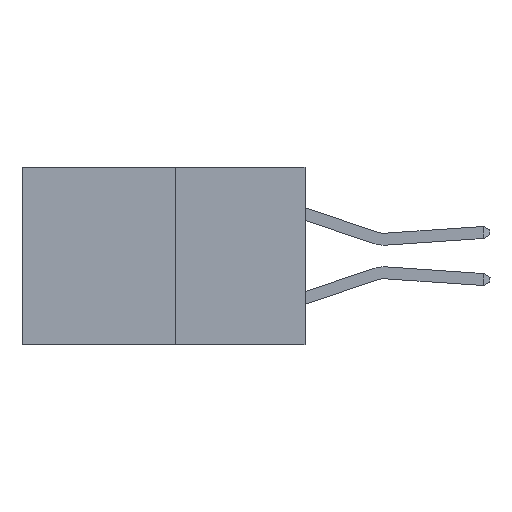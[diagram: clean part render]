
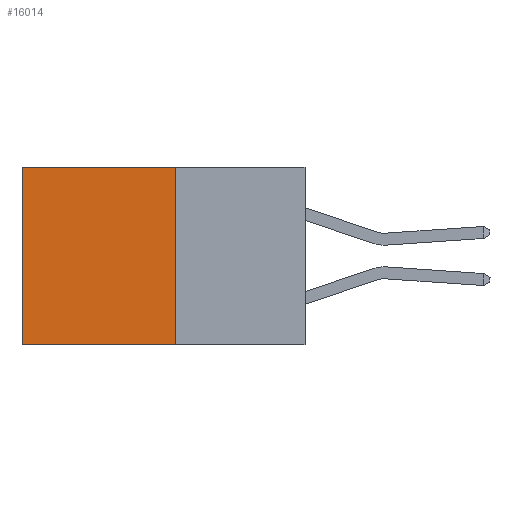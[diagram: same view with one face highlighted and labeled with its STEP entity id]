
A CAD part, left-side view. The second image highlights one B-rep face of the part: STEP entity #16014.
In plain terms, the highlighted planar face has unit normal (-1, 0, 0).
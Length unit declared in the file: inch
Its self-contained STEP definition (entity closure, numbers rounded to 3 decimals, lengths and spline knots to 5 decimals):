
#1238 = EDGE_LOOP ( 'NONE', ( #16327, #9316, #17948, #20871 ) ) ;
#1451 = PLANE ( 'NONE',  #13199 ) ;
#2006 = CARTESIAN_POINT ( 'NONE',  ( 0.277, 0.27, 0. ) ) ;
#3659 = CARTESIAN_POINT ( 'NONE',  ( 0.277, 0.27, 0. ) ) ;
#4166 = DIRECTION ( 'NONE',  ( 0., 1., 0. ) ) ;
#5233 = EDGE_CURVE ( 'NONE', #19410, #13453, #23947, .T. ) ;
#5755 = DIRECTION ( 'NONE',  ( 0., 1., 0. ) ) ;
#5861 = CARTESIAN_POINT ( 'NONE',  ( 0.277, 0.59, 0. ) ) ;
#6057 = CARTESIAN_POINT ( 'NONE',  ( 0.277, 0.27, -0.37 ) ) ;
#8040 = VECTOR ( 'NONE', #5755, 39.37008 ) ;
#9316 = ORIENTED_EDGE ( 'NONE', *, *, #25436, .F. ) ;
#9379 = DIRECTION ( 'NONE',  ( 0., 0., -1. ) ) ;
#9954 = VERTEX_POINT ( 'NONE', #2006 ) ;
#9957 = CARTESIAN_POINT ( 'NONE',  ( 0.277, 0.59, -0.37 ) ) ;
#10355 = CARTESIAN_POINT ( 'NONE',  ( 0.277, 0.27, -0.37 ) ) ;
#11150 = VERTEX_POINT ( 'NONE', #15870 ) ;
#13199 = AXIS2_PLACEMENT_3D ( 'NONE', #22018, #26175, #13968 ) ;
#13453 = VERTEX_POINT ( 'NONE', #15407 ) ;
#13968 = DIRECTION ( 'NONE',  ( 0., 0., -1. ) ) ;
#15407 = CARTESIAN_POINT ( 'NONE',  ( 0.277, 0.59, -0.37 ) ) ;
#15466 = VECTOR ( 'NONE', #18342, 39.37008 ) ;
#15870 = CARTESIAN_POINT ( 'NONE',  ( 0.277, 0.27, -0.37 ) ) ;
#16014 = ADVANCED_FACE ( 'NONE', ( #16869 ), #1451, .F. ) ;
#16327 = ORIENTED_EDGE ( 'NONE', *, *, #5233, .T. ) ;
#16869 = FACE_OUTER_BOUND ( 'NONE', #1238, .T. ) ;
#17948 = ORIENTED_EDGE ( 'NONE', *, *, #22401, .F. ) ;
#18342 = DIRECTION ( 'NONE',  ( 0., 0., -1. ) ) ;
#18517 = VECTOR ( 'NONE', #9379, 39.37008 ) ;
#18964 = LINE ( 'NONE', #10355, #23100 ) ;
#19410 = VERTEX_POINT ( 'NONE', #5861 ) ;
#20871 = ORIENTED_EDGE ( 'NONE', *, *, #22985, .T. ) ;
#22018 = CARTESIAN_POINT ( 'NONE',  ( 0.277, 0.27, -0.37 ) ) ;
#22401 = EDGE_CURVE ( 'NONE', #9954, #11150, #26293, .T. ) ;
#22985 = EDGE_CURVE ( 'NONE', #9954, #19410, #23694, .T. ) ;
#23100 = VECTOR ( 'NONE', #4166, 39.37008 ) ;
#23694 = LINE ( 'NONE', #3659, #8040 ) ;
#23947 = LINE ( 'NONE', #9957, #18517 ) ;
#25436 = EDGE_CURVE ( 'NONE', #11150, #13453, #18964, .T. ) ;
#26175 = DIRECTION ( 'NONE',  ( 1., 0., 0. ) ) ;
#26293 = LINE ( 'NONE', #6057, #15466 ) ;
